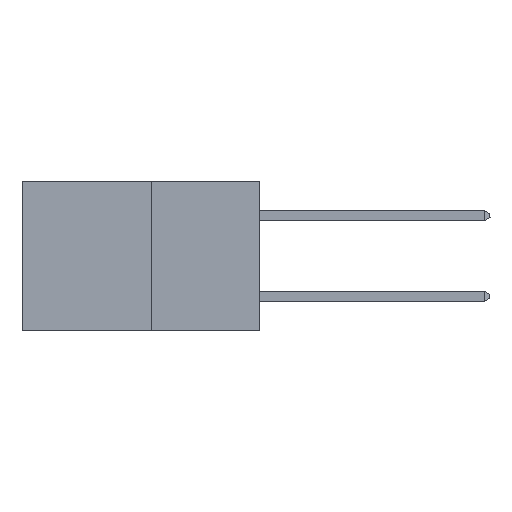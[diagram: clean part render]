
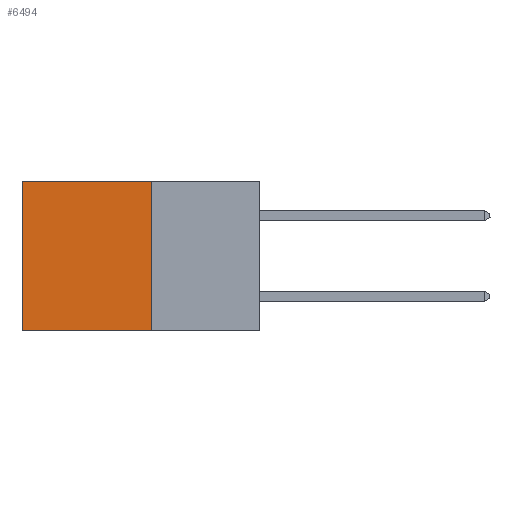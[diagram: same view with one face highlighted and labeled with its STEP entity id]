
A CAD part, left-side view. The second image highlights one B-rep face of the part: STEP entity #6494.
In plain terms, the highlighted planar face has unit normal (-1, 0, 0).
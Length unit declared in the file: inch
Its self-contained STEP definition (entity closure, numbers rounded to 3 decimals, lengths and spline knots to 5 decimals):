
#611 = ORIENTED_EDGE ( 'NONE', *, *, #8465, .T. ) ;
#2125 = FACE_OUTER_BOUND ( 'NONE', #20190, .T. ) ;
#3517 = EDGE_CURVE ( 'NONE', #10136, #19200, #5550, .T. ) ;
#4139 = VECTOR ( 'NONE', #10127, 39.37008 ) ;
#4408 = CARTESIAN_POINT ( 'NONE',  ( 0.277, 0.59, -0.37 ) ) ;
#5550 = LINE ( 'NONE', #27498, #25825 ) ;
#5723 = CARTESIAN_POINT ( 'NONE',  ( 0.277, 0.27, 0. ) ) ;
#6494 = ADVANCED_FACE ( 'NONE', ( #2125 ), #11907, .F. ) ;
#6978 = CARTESIAN_POINT ( 'NONE',  ( 0.277, 0.27, -0.37 ) ) ;
#8407 = VERTEX_POINT ( 'NONE', #25886 ) ;
#8465 = EDGE_CURVE ( 'NONE', #8407, #9932, #28081, .T. ) ;
#8967 = CARTESIAN_POINT ( 'NONE',  ( 0.277, 0.59, -0.37 ) ) ;
#9932 = VERTEX_POINT ( 'NONE', #8967 ) ;
#9975 = LINE ( 'NONE', #5723, #4139 ) ;
#10127 = DIRECTION ( 'NONE',  ( 0., 1., 0. ) ) ;
#10136 = VERTEX_POINT ( 'NONE', #10589 ) ;
#10434 = DIRECTION ( 'NONE',  ( 0., 0., -1. ) ) ;
#10589 = CARTESIAN_POINT ( 'NONE',  ( 0.277, 0.27, 0. ) ) ;
#11742 = AXIS2_PLACEMENT_3D ( 'NONE', #11997, #11815, #11751 ) ;
#11751 = DIRECTION ( 'NONE',  ( 0., 0., -1. ) ) ;
#11815 = DIRECTION ( 'NONE',  ( 1., 0., 0. ) ) ;
#11907 = PLANE ( 'NONE',  #11742 ) ;
#11997 = CARTESIAN_POINT ( 'NONE',  ( 0.277, 0.27, -0.37 ) ) ;
#12185 = LINE ( 'NONE', #6978, #17945 ) ;
#12366 = ORIENTED_EDGE ( 'NONE', *, *, #22433, .F. ) ;
#14844 = CARTESIAN_POINT ( 'NONE',  ( 0.277, 0.27, -0.37 ) ) ;
#16043 = VECTOR ( 'NONE', #19643, 39.37008 ) ;
#17945 = VECTOR ( 'NONE', #22133, 39.37008 ) ;
#18525 = EDGE_CURVE ( 'NONE', #10136, #8407, #9975, .T. ) ;
#19200 = VERTEX_POINT ( 'NONE', #14844 ) ;
#19643 = DIRECTION ( 'NONE',  ( 0., 0., -1. ) ) ;
#20190 = EDGE_LOOP ( 'NONE', ( #611, #12366, #23940, #21597 ) ) ;
#21597 = ORIENTED_EDGE ( 'NONE', *, *, #18525, .T. ) ;
#22133 = DIRECTION ( 'NONE',  ( 0., 1., 0. ) ) ;
#22433 = EDGE_CURVE ( 'NONE', #19200, #9932, #12185, .T. ) ;
#23940 = ORIENTED_EDGE ( 'NONE', *, *, #3517, .F. ) ;
#25825 = VECTOR ( 'NONE', #10434, 39.37008 ) ;
#25886 = CARTESIAN_POINT ( 'NONE',  ( 0.277, 0.59, 0. ) ) ;
#27498 = CARTESIAN_POINT ( 'NONE',  ( 0.277, 0.27, -0.37 ) ) ;
#28081 = LINE ( 'NONE', #4408, #16043 ) ;
